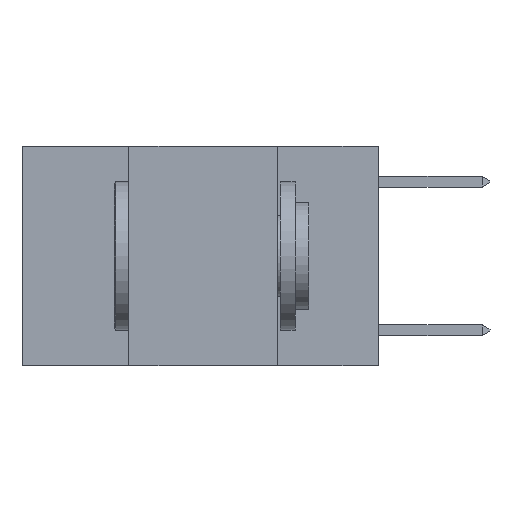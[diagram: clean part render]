
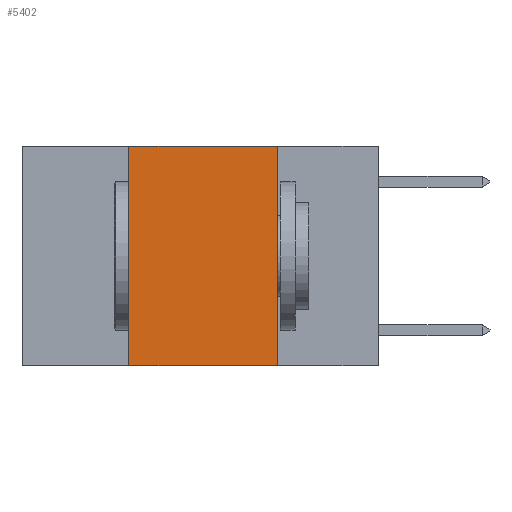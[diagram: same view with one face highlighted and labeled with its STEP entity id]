
A CAD part, left-side view. The second image highlights one B-rep face of the part: STEP entity #5402.
In plain terms, the highlighted planar face has unit normal (-1, 0, 0).
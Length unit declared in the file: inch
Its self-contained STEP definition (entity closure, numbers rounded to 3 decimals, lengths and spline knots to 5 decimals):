
#936 = VECTOR ( 'NONE', #3285, 39.37008 ) ;
#1068 = ORIENTED_EDGE ( 'NONE', *, *, #7106, .F. ) ;
#1344 = EDGE_CURVE ( 'NONE', #6239, #9829, #5399, .T. ) ;
#2317 = CARTESIAN_POINT ( 'NONE',  ( 0., 0.17, 0. ) ) ;
#2479 = EDGE_CURVE ( 'NONE', #3614, #6239, #5068, .T. ) ;
#2636 = FACE_OUTER_BOUND ( 'NONE', #13336, .T. ) ;
#2644 = VECTOR ( 'NONE', #2683, 39.37008 ) ;
#2683 = DIRECTION ( 'NONE',  ( 0., -1., 0. ) ) ;
#3285 = DIRECTION ( 'NONE',  ( 0., -1., 0. ) ) ;
#3511 = DIRECTION ( 'NONE',  ( 0., 0., -1. ) ) ;
#3614 = VERTEX_POINT ( 'NONE', #6272 ) ;
#3927 = CARTESIAN_POINT ( 'NONE',  ( 0., 0.17, 0. ) ) ;
#4584 = CARTESIAN_POINT ( 'NONE',  ( 0., 0.6, 0. ) ) ;
#5068 = LINE ( 'NONE', #10232, #12498 ) ;
#5399 = LINE ( 'NONE', #4584, #936 ) ;
#5402 = ADVANCED_FACE ( 'NONE', ( #2636 ), #12212, .F. ) ;
#5459 = CARTESIAN_POINT ( 'NONE',  ( 0., 0.6, -0.37 ) ) ;
#6239 = VERTEX_POINT ( 'NONE', #16235 ) ;
#6272 = CARTESIAN_POINT ( 'NONE',  ( 0., 0.42, -0.37 ) ) ;
#7106 = EDGE_CURVE ( 'NONE', #9829, #7795, #8892, .T. ) ;
#7530 = DIRECTION ( 'NONE',  ( 0., 0., 1. ) ) ;
#7619 = ORIENTED_EDGE ( 'NONE', *, *, #1344, .F. ) ;
#7795 = VERTEX_POINT ( 'NONE', #10327 ) ;
#8892 = LINE ( 'NONE', #3927, #16649 ) ;
#9829 = VERTEX_POINT ( 'NONE', #2317 ) ;
#9973 = ORIENTED_EDGE ( 'NONE', *, *, #2479, .F. ) ;
#10199 = ORIENTED_EDGE ( 'NONE', *, *, #13138, .T. ) ;
#10232 = CARTESIAN_POINT ( 'NONE',  ( 0., 0.42, 0. ) ) ;
#10327 = CARTESIAN_POINT ( 'NONE',  ( 0., 0.17, -0.37 ) ) ;
#10443 = DIRECTION ( 'NONE',  ( 0., 0., -1. ) ) ;
#10622 = DIRECTION ( 'NONE',  ( 1., 0., 0. ) ) ;
#12212 = PLANE ( 'NONE',  #13900 ) ;
#12498 = VECTOR ( 'NONE', #7530, 39.37008 ) ;
#13138 = EDGE_CURVE ( 'NONE', #3614, #7795, #13831, .T. ) ;
#13195 = CARTESIAN_POINT ( 'NONE',  ( 0., 0.6, 0. ) ) ;
#13336 = EDGE_LOOP ( 'NONE', ( #1068, #7619, #9973, #10199 ) ) ;
#13831 = LINE ( 'NONE', #5459, #2644 ) ;
#13900 = AXIS2_PLACEMENT_3D ( 'NONE', #13195, #10622, #10443 ) ;
#16235 = CARTESIAN_POINT ( 'NONE',  ( 0., 0.42, 0. ) ) ;
#16649 = VECTOR ( 'NONE', #3511, 39.37008 ) ;
